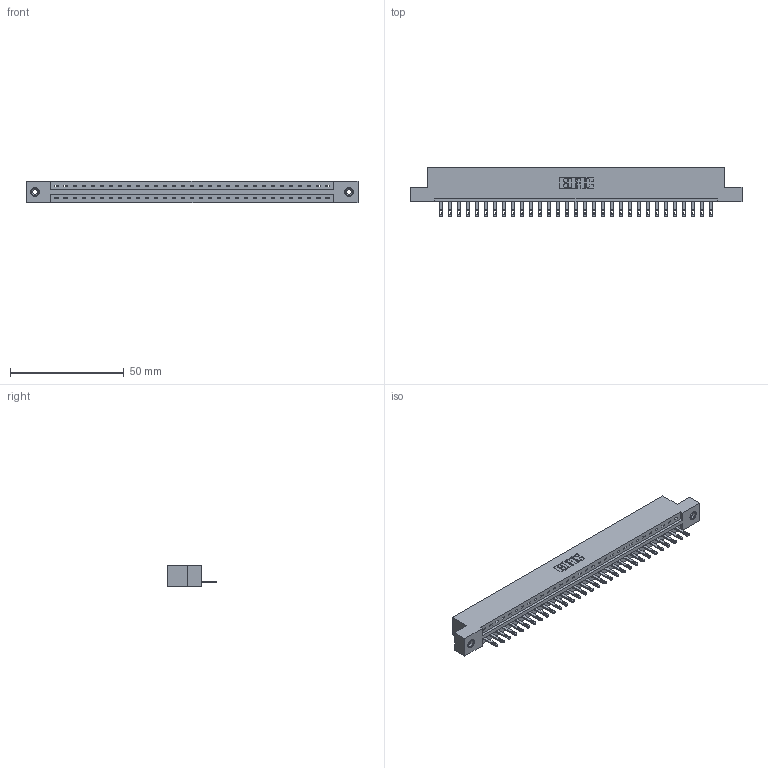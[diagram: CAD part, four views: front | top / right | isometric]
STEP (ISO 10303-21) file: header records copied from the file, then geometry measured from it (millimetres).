
FILE_DESCRIPTION (( 'STEP AP203' ), '1' );
FILE_NAME ('887-031-500-108.STEP', '2020-09-20T20:53:00', ( '' ), ( '' ), 'SwSTEP 2.0', 'SolidWorks 2020', '' );
FILE_SCHEMA (( 'CONFIG_CONTROL_DESIGN' ));
Length unit declared in the file: inch
Products named in the file (4): 345-292-001_345-293-100; 837 Part_Flush Mounting Lugs - 0.156 Dia-TI; 887-031-500-108; 345-250-001_345-250-003-102
Assembly tree (34 placements, depth 2):
  887-031-500-108
    837 Part_Flush Mounting Lugs - 0.156 Dia-TI
    345-292-001_345-293-100  x31
    345-250-001_345-250-003-102  x2
Bounding box: 145.85 x 21.85 x 9.4 mm (x, y, z)
Volume: 15033.3 mm3; surface area: 15575.8 mm2
Topology: 34 solids, 34 shells, 1972 faces, 6027 edges, 4010 vertices
Faces by surface type: plane 1342, cylinder 614, cone 12, torus 4
Entity records: 25582 total; most frequent: CARTESIAN_POINT 4434, ORIENTED_EDGE 4394, DIRECTION 3789, EDGE_CURVE 2197, LINE 2045, VECTOR 2045, VERTEX_POINT 1460, AXIS2_PLACEMENT_3D 872
